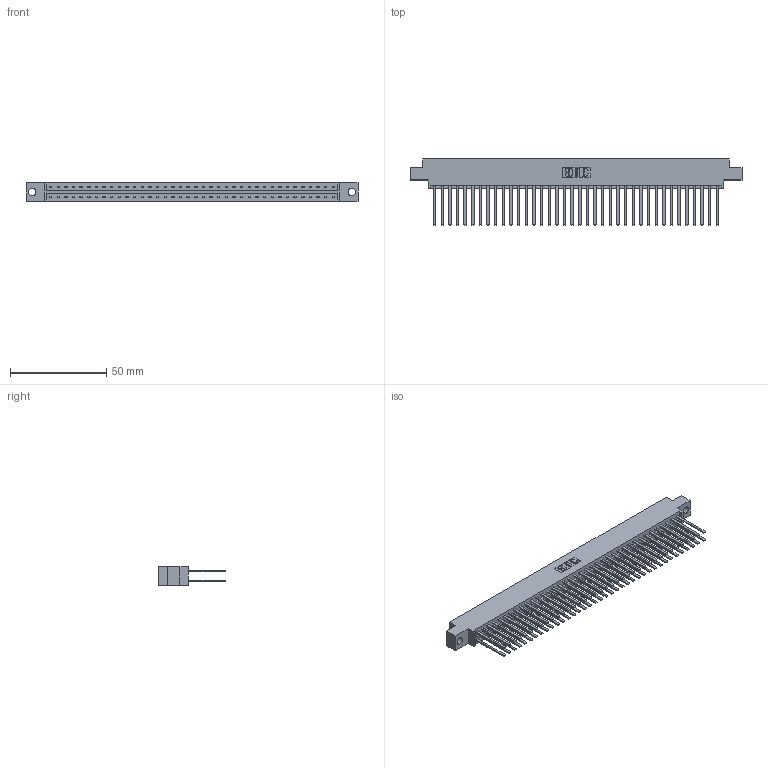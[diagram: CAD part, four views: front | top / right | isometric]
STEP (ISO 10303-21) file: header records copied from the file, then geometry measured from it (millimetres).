
FILE_DESCRIPTION (( 'STEP AP203' ), '1' );
FILE_NAME ('833-076-544-804.STEP', '2020-06-05T18:42:42', ( '' ), ( '' ), 'SwSTEP 2.0', 'SolidWorks 2020', '' );
FILE_SCHEMA (( 'CONFIG_CONTROL_DESIGN' ));
Length unit declared in the file: inch
Products named in the file (3): 833-076-544-804; 833 Part_Offset - .156 Dia - TH; 345-292-001_345-293-144
Assembly tree (77 placements, depth 2):
  833-076-544-804
    833 Part_Offset - .156 Dia - TH
    345-292-001_345-293-144  x76
Bounding box: 172.11 x 34.3 x 9.4 mm (x, y, z)
Volume: 18283.8 mm3; surface area: 25023.5 mm2
Topology: 77 solids, 77 shells, 3614 faces, 10735 edges, 7054 vertices
Faces by surface type: plane 2506, cylinder 1108
Entity records: 24915 total; most frequent: CARTESIAN_POINT 4134, ORIENTED_EDGE 4070, DIRECTION 3535, EDGE_CURVE 2035, VECTOR 1911, LINE 1911, VERTEX_POINT 1354, AXIS2_PLACEMENT_3D 812
